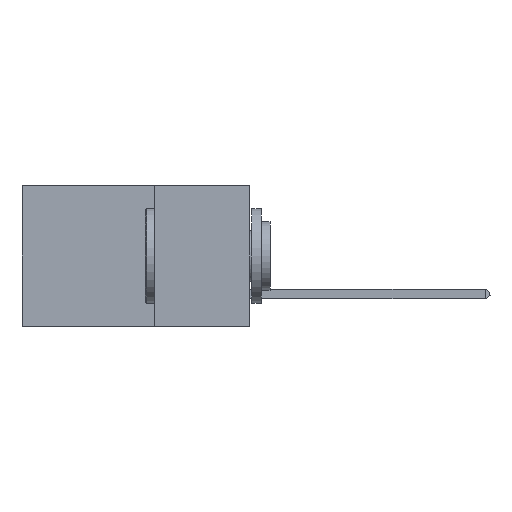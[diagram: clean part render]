
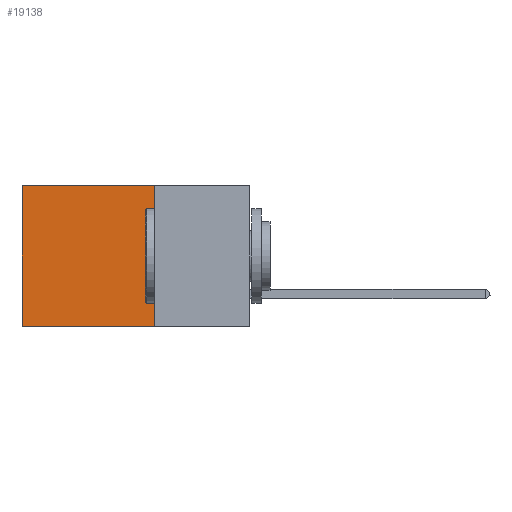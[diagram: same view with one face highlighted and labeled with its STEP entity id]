
A CAD part, left-side view. The second image highlights one B-rep face of the part: STEP entity #19138.
In plain terms, the highlighted planar face has unit normal (-1, 0, 0).
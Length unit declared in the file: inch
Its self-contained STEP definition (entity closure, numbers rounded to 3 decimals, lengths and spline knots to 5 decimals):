
#885 = VERTEX_POINT ( 'NONE', #34859 ) ;
#967 = VERTEX_POINT ( 'NONE', #3385 ) ;
#1918 = CARTESIAN_POINT ( 'NONE',  ( 0.2875, 0.6, -0.37 ) ) ;
#2566 = DIRECTION ( 'NONE',  ( 1., 0., 0. ) ) ;
#3385 = CARTESIAN_POINT ( 'NONE',  ( 0.2875, 0.25, -0.37 ) ) ;
#4904 = EDGE_CURVE ( 'NONE', #885, #32021, #30843, .T. ) ;
#6087 = FACE_OUTER_BOUND ( 'NONE', #19586, .T. ) ;
#7053 = EDGE_CURVE ( 'NONE', #967, #32021, #21611, .T. ) ;
#8843 = DIRECTION ( 'NONE',  ( 0., 0., -1. ) ) ;
#9745 = AXIS2_PLACEMENT_3D ( 'NONE', #19792, #2566, #24144 ) ;
#12535 = ORIENTED_EDGE ( 'NONE', *, *, #7053, .F. ) ;
#12778 = CARTESIAN_POINT ( 'NONE',  ( 0.2875, 0.6, 0. ) ) ;
#13150 = DIRECTION ( 'NONE',  ( 0., 0., -1. ) ) ;
#13582 = ORIENTED_EDGE ( 'NONE', *, *, #43651, .T. ) ;
#13586 = ORIENTED_EDGE ( 'NONE', *, *, #4904, .T. ) ;
#15102 = LINE ( 'NONE', #19175, #43592 ) ;
#17254 = VECTOR ( 'NONE', #32617, 39.37008 ) ;
#19138 = ADVANCED_FACE ( 'NONE', ( #6087 ), #19948, .F. ) ;
#19175 = CARTESIAN_POINT ( 'NONE',  ( 0.2875, 0.25, 0. ) ) ;
#19586 = EDGE_LOOP ( 'NONE', ( #13586, #12535, #23356, #13582 ) ) ;
#19792 = CARTESIAN_POINT ( 'NONE',  ( 0.2875, 0.25, 0. ) ) ;
#19948 = PLANE ( 'NONE',  #9745 ) ;
#21611 = LINE ( 'NONE', #28880, #17254 ) ;
#21779 = VECTOR ( 'NONE', #8843, 39.37008 ) ;
#22648 = VECTOR ( 'NONE', #13150, 39.37008 ) ;
#23356 = ORIENTED_EDGE ( 'NONE', *, *, #30326, .F. ) ;
#23685 = CARTESIAN_POINT ( 'NONE',  ( 0.2875, 0.25, 0. ) ) ;
#24144 = DIRECTION ( 'NONE',  ( 0., 0., -1. ) ) ;
#28880 = CARTESIAN_POINT ( 'NONE',  ( 0.2875, 0.25, -0.37 ) ) ;
#30326 = EDGE_CURVE ( 'NONE', #40526, #967, #31734, .T. ) ;
#30843 = LINE ( 'NONE', #12778, #21779 ) ;
#31734 = LINE ( 'NONE', #23685, #22648 ) ;
#32021 = VERTEX_POINT ( 'NONE', #1918 ) ;
#32617 = DIRECTION ( 'NONE',  ( 0., 1., 0. ) ) ;
#34859 = CARTESIAN_POINT ( 'NONE',  ( 0.2875, 0.6, 0. ) ) ;
#36199 = DIRECTION ( 'NONE',  ( 0., 1., 0. ) ) ;
#40526 = VERTEX_POINT ( 'NONE', #41668 ) ;
#41668 = CARTESIAN_POINT ( 'NONE',  ( 0.2875, 0.25, 0. ) ) ;
#43592 = VECTOR ( 'NONE', #36199, 39.37008 ) ;
#43651 = EDGE_CURVE ( 'NONE', #40526, #885, #15102, .T. ) ;
